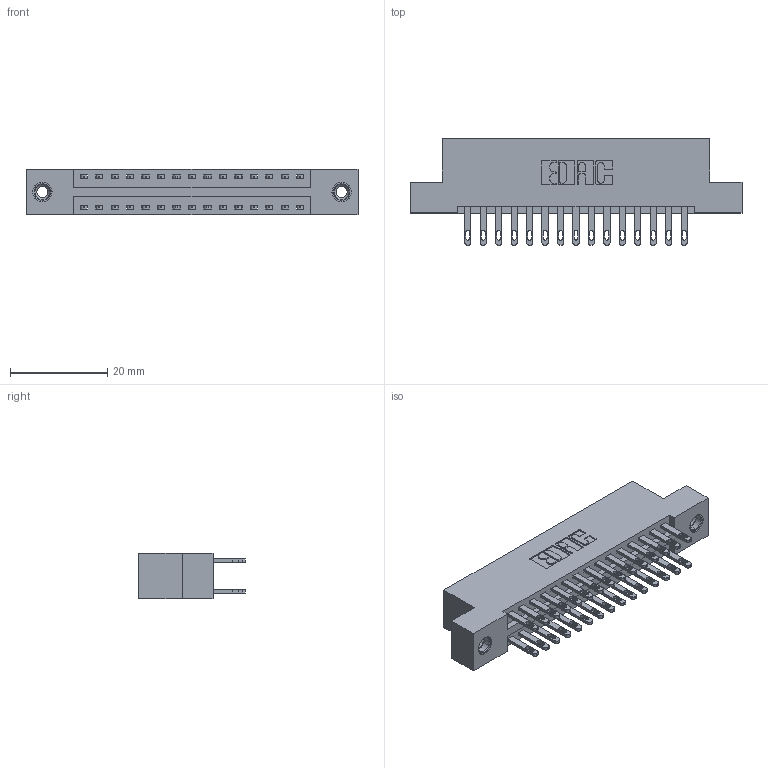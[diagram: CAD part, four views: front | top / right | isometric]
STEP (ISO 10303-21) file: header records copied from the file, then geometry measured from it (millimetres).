
FILE_DESCRIPTION (( 'STEP AP203' ), '1' );
FILE_NAME ('346-030-500-208.STEP', '2018-08-22T04:02:36', ( '' ), ( '' ), 'SwSTEP 2.0', 'SolidWorks 2016', '' );
FILE_SCHEMA (( 'CONFIG_CONTROL_DESIGN' ));
Length unit declared in the file: inch
Products named in the file (4): 346 Part_Flush Mounting Lugs - 0.156 Dia-TI; 345-292-001_345-293-100; 345-250-001_345-250-003-102; 346-030-500-208
Assembly tree (33 placements, depth 2):
  346-030-500-208
    346 Part_Flush Mounting Lugs - 0.156 Dia-TI
    345-292-001_345-293-100  x30
    345-250-001_345-250-003-102  x2
Bounding box: 68.2 x 21.84 x 9.4 mm (x, y, z)
Volume: 6525.7 mm3; surface area: 8879.7 mm2
Topology: 33 solids, 33 shells, 1622 faces, 4875 edges, 3242 vertices
Faces by surface type: plane 978, cylinder 628, cone 12, torus 4
Entity records: 14540 total; most frequent: CARTESIAN_POINT 2415, ORIENTED_EDGE 2342, DIRECTION 2209, EDGE_CURVE 1171, VECTOR 955, LINE 955, VERTEX_POINT 776, AXIS2_PLACEMENT_3D 627
